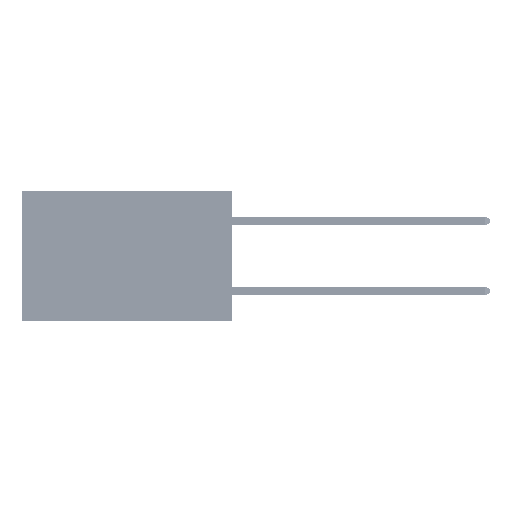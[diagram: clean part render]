
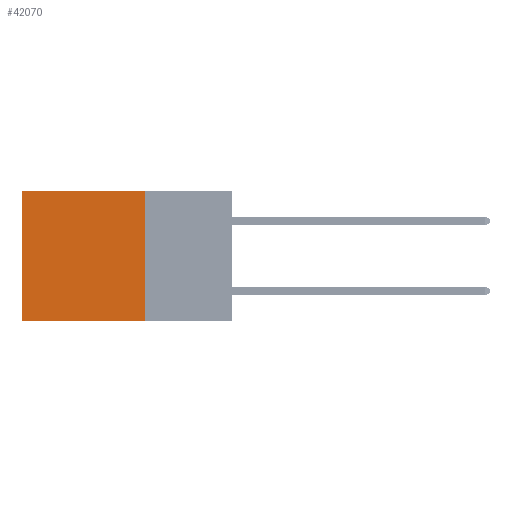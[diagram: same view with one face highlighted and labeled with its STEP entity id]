
A CAD part, left-side view. The second image highlights one B-rep face of the part: STEP entity #42070.
In plain terms, the highlighted planar face has unit normal (-1, 0, 0).
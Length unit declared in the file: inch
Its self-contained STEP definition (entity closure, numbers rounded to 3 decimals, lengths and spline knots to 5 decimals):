
#2986 = EDGE_CURVE ( 'NONE', #7555, #25863, #18982, .T. ) ;
#3003 = EDGE_CURVE ( 'NONE', #33272, #30854, #11409, .T. ) ;
#4643 = VECTOR ( 'NONE', #45152, 39.37008 ) ;
#5215 = AXIS2_PLACEMENT_3D ( 'NONE', #25957, #42184, #37481 ) ;
#6991 = CARTESIAN_POINT ( 'NONE',  ( 0.2875, 0.6, 0. ) ) ;
#7555 = VERTEX_POINT ( 'NONE', #41732 ) ;
#9591 = EDGE_CURVE ( 'NONE', #30854, #25863, #26853, .T. ) ;
#10280 = FACE_OUTER_BOUND ( 'NONE', #24786, .T. ) ;
#11169 = CARTESIAN_POINT ( 'NONE',  ( 0.2875, 0.6, -0.37 ) ) ;
#11409 = LINE ( 'NONE', #27087, #20138 ) ;
#18982 = LINE ( 'NONE', #43051, #40167 ) ;
#20138 = VECTOR ( 'NONE', #27346, 39.37008 ) ;
#20409 = VECTOR ( 'NONE', #50136, 39.37008 ) ;
#20994 = ORIENTED_EDGE ( 'NONE', *, *, #47370, .F. ) ;
#24786 = EDGE_LOOP ( 'NONE', ( #30375, #25037, #20994, #37947 ) ) ;
#25037 = ORIENTED_EDGE ( 'NONE', *, *, #2986, .F. ) ;
#25863 = VERTEX_POINT ( 'NONE', #11169 ) ;
#25957 = CARTESIAN_POINT ( 'NONE',  ( 0.2875, 0.25, 0. ) ) ;
#26215 = PLANE ( 'NONE',  #5215 ) ;
#26445 = CARTESIAN_POINT ( 'NONE',  ( 0.2875, 0.6, 0. ) ) ;
#26853 = LINE ( 'NONE', #6991, #20409 ) ;
#27087 = CARTESIAN_POINT ( 'NONE',  ( 0.2875, 0.25, 0. ) ) ;
#27346 = DIRECTION ( 'NONE',  ( 0., 1., 0. ) ) ;
#29191 = CARTESIAN_POINT ( 'NONE',  ( 0.2875, 0.25, 0. ) ) ;
#30375 = ORIENTED_EDGE ( 'NONE', *, *, #9591, .T. ) ;
#30854 = VERTEX_POINT ( 'NONE', #26445 ) ;
#33272 = VERTEX_POINT ( 'NONE', #48580 ) ;
#37481 = DIRECTION ( 'NONE',  ( 0., 0., -1. ) ) ;
#37565 = LINE ( 'NONE', #29191, #4643 ) ;
#37947 = ORIENTED_EDGE ( 'NONE', *, *, #3003, .T. ) ;
#40167 = VECTOR ( 'NONE', #51140, 39.37008 ) ;
#41732 = CARTESIAN_POINT ( 'NONE',  ( 0.2875, 0.25, -0.37 ) ) ;
#42070 = ADVANCED_FACE ( 'NONE', ( #10280 ), #26215, .F. ) ;
#42184 = DIRECTION ( 'NONE',  ( 1., 0., 0. ) ) ;
#43051 = CARTESIAN_POINT ( 'NONE',  ( 0.2875, 0.25, -0.37 ) ) ;
#45152 = DIRECTION ( 'NONE',  ( 0., 0., -1. ) ) ;
#47370 = EDGE_CURVE ( 'NONE', #33272, #7555, #37565, .T. ) ;
#48580 = CARTESIAN_POINT ( 'NONE',  ( 0.2875, 0.25, 0. ) ) ;
#50136 = DIRECTION ( 'NONE',  ( 0., 0., -1. ) ) ;
#51140 = DIRECTION ( 'NONE',  ( 0., 1., 0. ) ) ;
